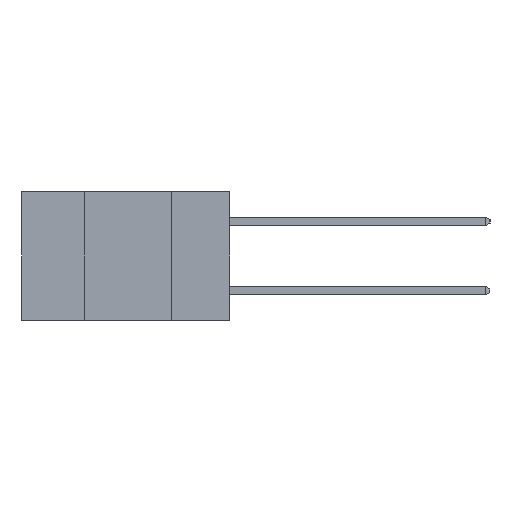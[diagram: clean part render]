
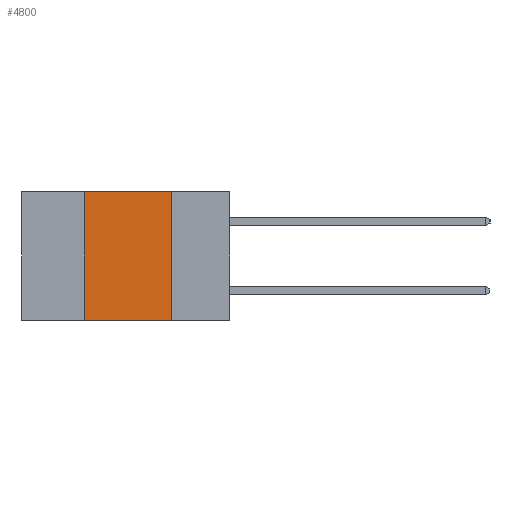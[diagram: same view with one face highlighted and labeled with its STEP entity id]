
A CAD part, left-side view. The second image highlights one B-rep face of the part: STEP entity #4800.
In plain terms, the highlighted planar face has unit normal (-1, 0, 0).
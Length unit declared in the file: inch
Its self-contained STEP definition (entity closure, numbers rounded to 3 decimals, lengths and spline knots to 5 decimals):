
#1955 = VECTOR ( 'NONE', #20528, 39.37008 ) ;
#2608 = CARTESIAN_POINT ( 'NONE',  ( 0., 0.17, -0.37 ) ) ;
#3300 = LINE ( 'NONE', #22721, #14040 ) ;
#4073 = EDGE_CURVE ( 'NONE', #13728, #16618, #3300, .T. ) ;
#4744 = EDGE_LOOP ( 'NONE', ( #20650, #9438, #23301, #9149 ) ) ;
#4767 = DIRECTION ( 'NONE',  ( 0., 0., -1. ) ) ;
#4800 = ADVANCED_FACE ( 'NONE', ( #8655 ), #9192, .F. ) ;
#5292 = DIRECTION ( 'NONE',  ( 0., -1., 0. ) ) ;
#5368 = LINE ( 'NONE', #11674, #16032 ) ;
#8655 = FACE_OUTER_BOUND ( 'NONE', #4744, .T. ) ;
#9095 = DIRECTION ( 'NONE',  ( 0., 0., -1. ) ) ;
#9118 = DIRECTION ( 'NONE',  ( 1., 0., 0. ) ) ;
#9149 = ORIENTED_EDGE ( 'NONE', *, *, #17876, .T. ) ;
#9152 = CARTESIAN_POINT ( 'NONE',  ( 0., 0.6, 0. ) ) ;
#9192 = PLANE ( 'NONE',  #11801 ) ;
#9438 = ORIENTED_EDGE ( 'NONE', *, *, #22408, .F. ) ;
#10445 = CARTESIAN_POINT ( 'NONE',  ( 0., 0.42, -0.37 ) ) ;
#11188 = CARTESIAN_POINT ( 'NONE',  ( 0., 0.17, -0.37 ) ) ;
#11674 = CARTESIAN_POINT ( 'NONE',  ( 0., 0.6, 0. ) ) ;
#11801 = AXIS2_PLACEMENT_3D ( 'NONE', #9152, #9118, #9095 ) ;
#13728 = VERTEX_POINT ( 'NONE', #10445 ) ;
#14008 = LINE ( 'NONE', #14221, #1955 ) ;
#14040 = VECTOR ( 'NONE', #22371, 39.37008 ) ;
#14221 = CARTESIAN_POINT ( 'NONE',  ( 0., 0.6, -0.37 ) ) ;
#15313 = LINE ( 'NONE', #2608, #20840 ) ;
#16032 = VECTOR ( 'NONE', #5292, 39.37008 ) ;
#16618 = VERTEX_POINT ( 'NONE', #21583 ) ;
#17876 = EDGE_CURVE ( 'NONE', #13728, #22914, #14008, .T. ) ;
#18239 = EDGE_CURVE ( 'NONE', #21038, #22914, #15313, .T. ) ;
#20528 = DIRECTION ( 'NONE',  ( 0., -1., 0. ) ) ;
#20650 = ORIENTED_EDGE ( 'NONE', *, *, #18239, .F. ) ;
#20840 = VECTOR ( 'NONE', #4767, 39.37008 ) ;
#21038 = VERTEX_POINT ( 'NONE', #24091 ) ;
#21583 = CARTESIAN_POINT ( 'NONE',  ( 0., 0.42, 0. ) ) ;
#22371 = DIRECTION ( 'NONE',  ( 0., 0., 1. ) ) ;
#22408 = EDGE_CURVE ( 'NONE', #16618, #21038, #5368, .T. ) ;
#22721 = CARTESIAN_POINT ( 'NONE',  ( 0., 0.42, -0.37 ) ) ;
#22914 = VERTEX_POINT ( 'NONE', #11188 ) ;
#23301 = ORIENTED_EDGE ( 'NONE', *, *, #4073, .F. ) ;
#24091 = CARTESIAN_POINT ( 'NONE',  ( 0., 0.17, 0. ) ) ;
